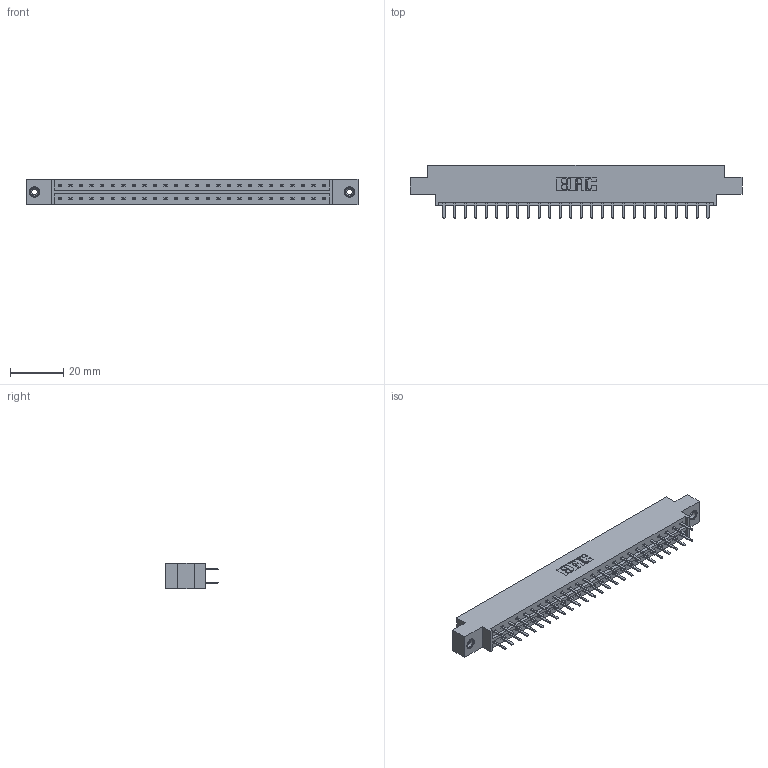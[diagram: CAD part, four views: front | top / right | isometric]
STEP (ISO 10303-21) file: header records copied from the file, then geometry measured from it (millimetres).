
FILE_DESCRIPTION (( 'STEP AP203' ), '1' );
FILE_NAME ('833-052-520-808.STEP', '2020-06-04T18:45:19', ( '' ), ( '' ), 'SwSTEP 2.0', 'SolidWorks 2020', '' );
FILE_SCHEMA (( 'CONFIG_CONTROL_DESIGN' ));
Length unit declared in the file: inch
Products named in the file (4): 345-292-001_345-293-120; 833 Part_Offset - .156 Dia - TI; 345-250-001_345-250-003-102; 833-052-520-808
Assembly tree (55 placements, depth 2):
  833-052-520-808
    833 Part_Offset - .156 Dia - TI
    345-292-001_345-293-120  x52
    345-250-001_345-250-003-102  x2
Bounding box: 124.56 x 20.02 x 9.4 mm (x, y, z)
Volume: 12310.2 mm3; surface area: 14563.9 mm2
Topology: 55 solids, 55 shells, 3090 faces, 8935 edges, 5810 vertices
Faces by surface type: plane 2082, cylinder 992, cone 12, torus 4
Entity records: 20228 total; most frequent: CARTESIAN_POINT 3369, ORIENTED_EDGE 3286, DIRECTION 2925, EDGE_CURVE 1643, LINE 1491, VECTOR 1491, VERTEX_POINT 1088, AXIS2_PLACEMENT_3D 717
